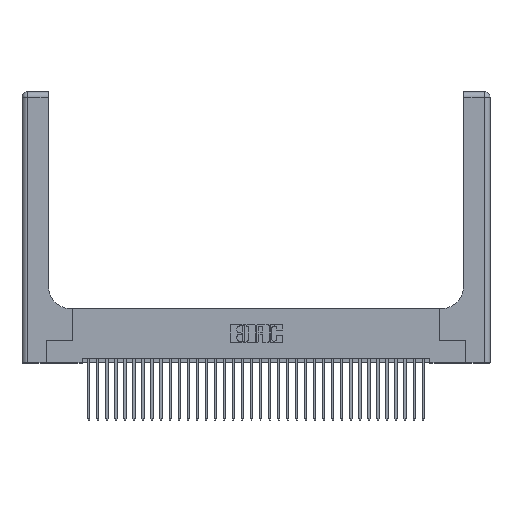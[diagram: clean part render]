
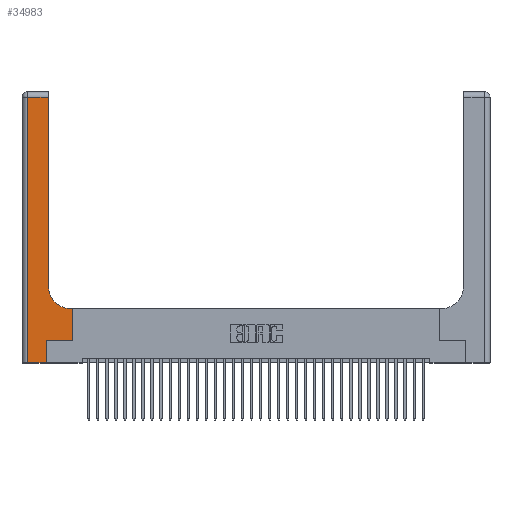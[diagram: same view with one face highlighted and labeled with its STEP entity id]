
A CAD part, top view. The second image highlights one B-rep face of the part: STEP entity #34983.
In plain terms, the highlighted planar face has unit normal (0, 0, 1).
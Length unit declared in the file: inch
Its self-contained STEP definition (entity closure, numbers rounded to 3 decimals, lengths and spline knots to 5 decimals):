
#703 = ORIENTED_EDGE ( 'NONE', *, *, #1510, .T. ) ;
#1444 = DIRECTION ( 'NONE',  ( -1., 0., 0. ) ) ;
#1510 = EDGE_CURVE ( 'NONE', #21174, #30310, #17994, .T. ) ;
#1591 = DIRECTION ( 'NONE',  ( 0., 1., 0. ) ) ;
#2941 = VECTOR ( 'NONE', #7214, 39.37008 ) ;
#3280 = VECTOR ( 'NONE', #23927, 39.37008 ) ;
#3503 = CARTESIAN_POINT ( 'NONE',  ( 0.2915, 2.94, 0.37 ) ) ;
#3651 = VERTEX_POINT ( 'NONE', #3503 ) ;
#3781 = CARTESIAN_POINT ( 'NONE',  ( 0.269, 0., 0.37 ) ) ;
#4314 = CARTESIAN_POINT ( 'NONE',  ( 0.5415, 0.85, 0.37 ) ) ;
#4353 = CARTESIAN_POINT ( 'NONE',  ( 0.06, 3., 0.37 ) ) ;
#5205 = FACE_OUTER_BOUND ( 'NONE', #11518, .T. ) ;
#5694 = CARTESIAN_POINT ( 'NONE',  ( 0.06, 0., 0.37 ) ) ;
#6038 = ORIENTED_EDGE ( 'NONE', *, *, #34954, .T. ) ;
#6059 = VERTEX_POINT ( 'NONE', #24325 ) ;
#6094 = VECTOR ( 'NONE', #1591, 39.37008 ) ;
#7040 = LINE ( 'NONE', #34299, #30602 ) ;
#7171 = DIRECTION ( 'NONE',  ( 1., 0., 0. ) ) ;
#7214 = DIRECTION ( 'NONE',  ( 0., -1., 0. ) ) ;
#7997 = LINE ( 'NONE', #35477, #15306 ) ;
#8083 = DIRECTION ( 'NONE',  ( 1., 0., 0. ) ) ;
#8775 = DIRECTION ( 'NONE',  ( 1., 0., 0. ) ) ;
#9277 = EDGE_CURVE ( 'NONE', #30310, #28722, #7040, .T. ) ;
#9580 = EDGE_CURVE ( 'NONE', #18745, #21174, #7997, .T. ) ;
#9927 = CARTESIAN_POINT ( 'NONE',  ( 0.5415, 0.6, 0.37 ) ) ;
#10019 = CARTESIAN_POINT ( 'NONE',  ( 0., 3., 0.37 ) ) ;
#10134 = PLANE ( 'NONE',  #34714 ) ;
#10341 = LINE ( 'NONE', #4353, #2941 ) ;
#11045 = DIRECTION ( 'NONE',  ( -1., 0., 0. ) ) ;
#11518 = EDGE_LOOP ( 'NONE', ( #28472, #26343, #22322, #20565, #6038, #34624, #703, #15419, #23019 ) ) ;
#12893 = DIRECTION ( 'NONE',  ( 0., 0., -1. ) ) ;
#13464 = LINE ( 'NONE', #3781, #6094 ) ;
#14775 = EDGE_CURVE ( 'NONE', #3651, #25406, #29488, .T. ) ;
#14789 = CARTESIAN_POINT ( 'NONE',  ( 0.269, 0.25, 0.37 ) ) ;
#15306 = VECTOR ( 'NONE', #8083, 39.37008 ) ;
#15419 = ORIENTED_EDGE ( 'NONE', *, *, #9277, .T. ) ;
#17139 = AXIS2_PLACEMENT_3D ( 'NONE', #4314, #23597, #7171 ) ;
#17994 = LINE ( 'NONE', #34679, #3280 ) ;
#18745 = VERTEX_POINT ( 'NONE', #14789 ) ;
#20018 = LINE ( 'NONE', #27933, #26452 ) ;
#20205 = VECTOR ( 'NONE', #24887, 39.37008 ) ;
#20565 = ORIENTED_EDGE ( 'NONE', *, *, #23423, .T. ) ;
#20997 = EDGE_CURVE ( 'NONE', #25406, #28409, #10341, .T. ) ;
#21067 = LINE ( 'NONE', #30334, #20205 ) ;
#21174 = VERTEX_POINT ( 'NONE', #32429 ) ;
#22322 = ORIENTED_EDGE ( 'NONE', *, *, #20997, .T. ) ;
#22895 = CARTESIAN_POINT ( 'NONE',  ( 0.5585, 0.6, 0.37 ) ) ;
#23011 = CIRCLE ( 'NONE', #17139, 0.25 ) ;
#23019 = ORIENTED_EDGE ( 'NONE', *, *, #23555, .T. ) ;
#23423 = EDGE_CURVE ( 'NONE', #28409, #6059, #20018, .T. ) ;
#23555 = EDGE_CURVE ( 'NONE', #28722, #31019, #23011, .T. ) ;
#23597 = DIRECTION ( 'NONE',  ( 0., 0., -1. ) ) ;
#23927 = DIRECTION ( 'NONE',  ( 0., 1., 0. ) ) ;
#24325 = CARTESIAN_POINT ( 'NONE',  ( 0.269, 0., 0.37 ) ) ;
#24887 = DIRECTION ( 'NONE',  ( 0., 1., 0. ) ) ;
#25406 = VERTEX_POINT ( 'NONE', #28361 ) ;
#26343 = ORIENTED_EDGE ( 'NONE', *, *, #14775, .T. ) ;
#26452 = VECTOR ( 'NONE', #8775, 39.37008 ) ;
#27933 = CARTESIAN_POINT ( 'NONE',  ( 0., 0., 0.37 ) ) ;
#28361 = CARTESIAN_POINT ( 'NONE',  ( 0.06, 2.94, 0.37 ) ) ;
#28409 = VERTEX_POINT ( 'NONE', #5694 ) ;
#28472 = ORIENTED_EDGE ( 'NONE', *, *, #35252, .T. ) ;
#28647 = VECTOR ( 'NONE', #11045, 39.37008 ) ;
#28722 = VERTEX_POINT ( 'NONE', #9927 ) ;
#29488 = LINE ( 'NONE', #35468, #28647 ) ;
#30310 = VERTEX_POINT ( 'NONE', #22895 ) ;
#30334 = CARTESIAN_POINT ( 'NONE',  ( 0.2915, 3., 0.37 ) ) ;
#30602 = VECTOR ( 'NONE', #1444, 39.37008 ) ;
#31019 = VERTEX_POINT ( 'NONE', #34444 ) ;
#32001 = DIRECTION ( 'NONE',  ( -1., 0., 0. ) ) ;
#32429 = CARTESIAN_POINT ( 'NONE',  ( 0.5585, 0.25, 0.37 ) ) ;
#34299 = CARTESIAN_POINT ( 'NONE',  ( 0.2915, 0.6, 0.37 ) ) ;
#34444 = CARTESIAN_POINT ( 'NONE',  ( 0.2915, 0.85, 0.37 ) ) ;
#34624 = ORIENTED_EDGE ( 'NONE', *, *, #9580, .T. ) ;
#34679 = CARTESIAN_POINT ( 'NONE',  ( 0.5585, 0.25, 0.37 ) ) ;
#34714 = AXIS2_PLACEMENT_3D ( 'NONE', #10019, #12893, #32001 ) ;
#34954 = EDGE_CURVE ( 'NONE', #6059, #18745, #13464, .T. ) ;
#34983 = ADVANCED_FACE ( 'NONE', ( #5205 ), #10134, .F. ) ;
#35252 = EDGE_CURVE ( 'NONE', #31019, #3651, #21067, .T. ) ;
#35468 = CARTESIAN_POINT ( 'NONE',  ( 0., 2.94, 0.37 ) ) ;
#35477 = CARTESIAN_POINT ( 'NONE',  ( 0.269, 0.25, 0.37 ) ) ;
